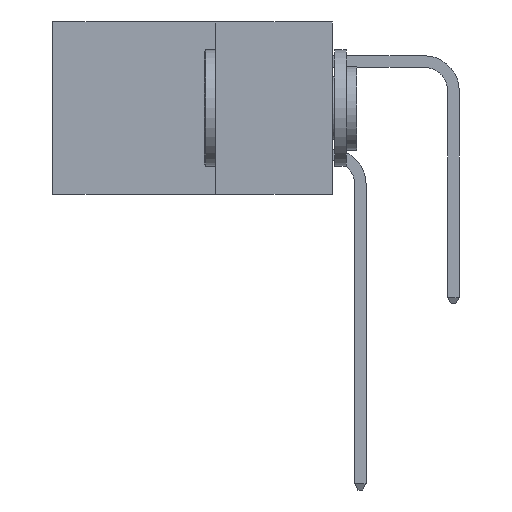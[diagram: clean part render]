
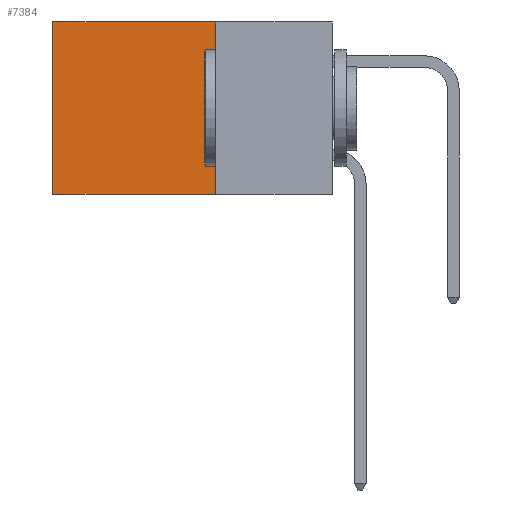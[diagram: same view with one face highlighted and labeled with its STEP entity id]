
A CAD part, left-side view. The second image highlights one B-rep face of the part: STEP entity #7384.
In plain terms, the highlighted planar face has unit normal (-1, 0, 0).
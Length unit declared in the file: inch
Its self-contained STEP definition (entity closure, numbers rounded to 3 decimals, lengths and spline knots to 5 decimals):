
#100 = VERTEX_POINT ( 'NONE', #23634 ) ;
#174 = DIRECTION ( 'NONE',  ( 0., 1., 0. ) ) ;
#276 = CARTESIAN_POINT ( 'NONE',  ( 0.2615, 0.25, 0. ) ) ;
#1719 = EDGE_LOOP ( 'NONE', ( #17237, #4792, #10089, #20703 ) ) ;
#2803 = CARTESIAN_POINT ( 'NONE',  ( 0.2615, 0.25, -0.37 ) ) ;
#2996 = VERTEX_POINT ( 'NONE', #23483 ) ;
#3331 = VECTOR ( 'NONE', #17585, 39.37008 ) ;
#4304 = EDGE_CURVE ( 'NONE', #100, #10774, #13916, .T. ) ;
#4361 = PLANE ( 'NONE',  #5464 ) ;
#4405 = DIRECTION ( 'NONE',  ( 0., 0., -1. ) ) ;
#4541 = CARTESIAN_POINT ( 'NONE',  ( 0.2615, 0.6, -0.37 ) ) ;
#4792 = ORIENTED_EDGE ( 'NONE', *, *, #22023, .F. ) ;
#5198 = EDGE_CURVE ( 'NONE', #2996, #100, #19842, .T. ) ;
#5464 = AXIS2_PLACEMENT_3D ( 'NONE', #20726, #17216, #6257 ) ;
#6257 = DIRECTION ( 'NONE',  ( 0., 0., -1. ) ) ;
#7384 = ADVANCED_FACE ( 'NONE', ( #14068 ), #4361, .F. ) ;
#8698 = DIRECTION ( 'NONE',  ( 0., 0., -1. ) ) ;
#9079 = VECTOR ( 'NONE', #4405, 39.37008 ) ;
#9436 = VECTOR ( 'NONE', #8698, 39.37008 ) ;
#10089 = ORIENTED_EDGE ( 'NONE', *, *, #23311, .F. ) ;
#10774 = VERTEX_POINT ( 'NONE', #23499 ) ;
#11320 = VECTOR ( 'NONE', #174, 39.37008 ) ;
#13485 = CARTESIAN_POINT ( 'NONE',  ( 0.2615, 0.25, -0.37 ) ) ;
#13916 = LINE ( 'NONE', #4541, #9079 ) ;
#14068 = FACE_OUTER_BOUND ( 'NONE', #1719, .T. ) ;
#17216 = DIRECTION ( 'NONE',  ( 1., 0., 0. ) ) ;
#17237 = ORIENTED_EDGE ( 'NONE', *, *, #4304, .T. ) ;
#17585 = DIRECTION ( 'NONE',  ( 0., 1., 0. ) ) ;
#17638 = VERTEX_POINT ( 'NONE', #13485 ) ;
#17980 = LINE ( 'NONE', #19604, #9436 ) ;
#19604 = CARTESIAN_POINT ( 'NONE',  ( 0.2615, 0.25, -0.37 ) ) ;
#19842 = LINE ( 'NONE', #276, #11320 ) ;
#20703 = ORIENTED_EDGE ( 'NONE', *, *, #5198, .T. ) ;
#20726 = CARTESIAN_POINT ( 'NONE',  ( 0.2615, 0.25, -0.37 ) ) ;
#22023 = EDGE_CURVE ( 'NONE', #17638, #10774, #22762, .T. ) ;
#22762 = LINE ( 'NONE', #2803, #3331 ) ;
#23311 = EDGE_CURVE ( 'NONE', #2996, #17638, #17980, .T. ) ;
#23483 = CARTESIAN_POINT ( 'NONE',  ( 0.2615, 0.25, 0. ) ) ;
#23499 = CARTESIAN_POINT ( 'NONE',  ( 0.2615, 0.6, -0.37 ) ) ;
#23634 = CARTESIAN_POINT ( 'NONE',  ( 0.2615, 0.6, 0. ) ) ;
